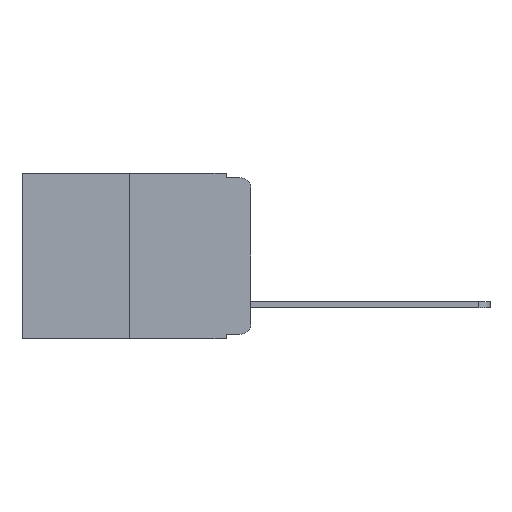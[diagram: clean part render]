
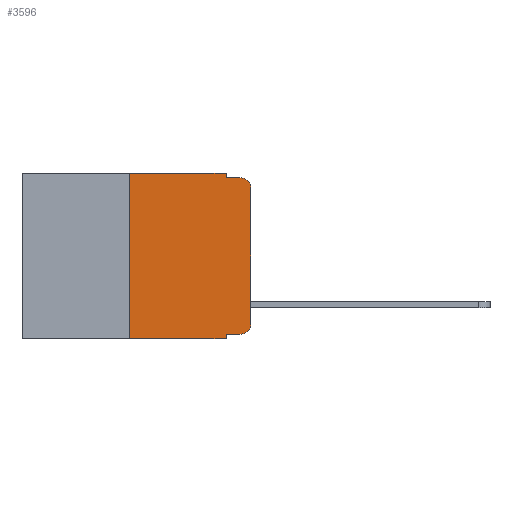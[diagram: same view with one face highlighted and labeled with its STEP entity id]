
A CAD part, left-side view. The second image highlights one B-rep face of the part: STEP entity #3596.
In plain terms, the highlighted planar face has unit normal (-1, 0, 0).
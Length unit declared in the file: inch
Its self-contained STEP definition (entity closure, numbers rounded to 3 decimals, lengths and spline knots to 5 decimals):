
#17 = CIRCLE ( 'NONE', #7517, 0.02 ) ;
#153 = CARTESIAN_POINT ( 'NONE',  ( 0., 0.051, -0.333 ) ) ;
#164 = CARTESIAN_POINT ( 'NONE',  ( 0., 0.473, 0. ) ) ;
#317 = EDGE_CURVE ( 'NONE', #16053, #17197, #1806, .T. ) ;
#400 = DIRECTION ( 'NONE',  ( -1., 0., 0. ) ) ;
#474 = EDGE_CURVE ( 'NONE', #8858, #903, #11412, .T. ) ;
#492 = CARTESIAN_POINT ( 'NONE',  ( 0., 0.051, -0.01 ) ) ;
#643 = VERTEX_POINT ( 'NONE', #5069 ) ;
#694 = CARTESIAN_POINT ( 'NONE',  ( 0., 0., 0. ) ) ;
#903 = VERTEX_POINT ( 'NONE', #4317 ) ;
#1048 = LINE ( 'NONE', #9050, #5649 ) ;
#1276 = EDGE_CURVE ( 'NONE', #903, #6998, #17, .T. ) ;
#1806 = LINE ( 'NONE', #12466, #5091 ) ;
#1963 = VECTOR ( 'NONE', #3531, 39.37008 ) ;
#2827 = ORIENTED_EDGE ( 'NONE', *, *, #474, .T. ) ;
#2914 = CARTESIAN_POINT ( 'NONE',  ( 0., 0.051, 0. ) ) ;
#3210 = DIRECTION ( 'NONE',  ( 0., 0., -1. ) ) ;
#3531 = DIRECTION ( 'NONE',  ( 0., 0., -1. ) ) ;
#3596 = ADVANCED_FACE ( 'NONE', ( #5192 ), #17017, .F. ) ;
#4317 = CARTESIAN_POINT ( 'NONE',  ( 0., 0., -0.03 ) ) ;
#4720 = ORIENTED_EDGE ( 'NONE', *, *, #8834, .T. ) ;
#4814 = CARTESIAN_POINT ( 'NONE',  ( 0., 0.02, -0.01 ) ) ;
#5069 = CARTESIAN_POINT ( 'NONE',  ( 0., 0.02, -0.333 ) ) ;
#5091 = VECTOR ( 'NONE', #14160, 39.37008 ) ;
#5192 = FACE_OUTER_BOUND ( 'NONE', #8830, .T. ) ;
#5333 = EDGE_CURVE ( 'NONE', #11239, #12072, #12685, .T. ) ;
#5520 = CARTESIAN_POINT ( 'NONE',  ( 0., 0.25, 0. ) ) ;
#5553 = VERTEX_POINT ( 'NONE', #153 ) ;
#5649 = VECTOR ( 'NONE', #6195, 39.37008 ) ;
#5858 = DIRECTION ( 'NONE',  ( 1., 0., 0. ) ) ;
#6097 = DIRECTION ( 'NONE',  ( 0., 0., 1. ) ) ;
#6195 = DIRECTION ( 'NONE',  ( 0., 0., -1. ) ) ;
#6376 = CIRCLE ( 'NONE', #9306, 0.02 ) ;
#6530 = EDGE_CURVE ( 'NONE', #5553, #17197, #1048, .T. ) ;
#6680 = VECTOR ( 'NONE', #7346, 39.37008 ) ;
#6871 = LINE ( 'NONE', #9982, #10804 ) ;
#6998 = VERTEX_POINT ( 'NONE', #4814 ) ;
#7221 = DIRECTION ( 'NONE',  ( 0., -1., 0. ) ) ;
#7275 = LINE ( 'NONE', #15207, #14508 ) ;
#7346 = DIRECTION ( 'NONE',  ( 0., -1., 0. ) ) ;
#7517 = AXIS2_PLACEMENT_3D ( 'NONE', #10187, #400, #3210 ) ;
#7597 = EDGE_CURVE ( 'NONE', #16053, #17313, #16533, .T. ) ;
#8536 = DIRECTION ( 'NONE',  ( 0., 0., -1. ) ) ;
#8585 = DIRECTION ( 'NONE',  ( 0., 0., -1. ) ) ;
#8830 = EDGE_LOOP ( 'NONE', ( #2827, #12749, #13470, #10991, #16631, #11613, #12989, #10913, #4720, #17436 ) ) ;
#8834 = EDGE_CURVE ( 'NONE', #5553, #643, #7275, .T. ) ;
#8858 = VERTEX_POINT ( 'NONE', #12462 ) ;
#9050 = CARTESIAN_POINT ( 'NONE',  ( 0., 0.051, 0. ) ) ;
#9155 = CARTESIAN_POINT ( 'NONE',  ( 0., 0.051, 0. ) ) ;
#9306 = AXIS2_PLACEMENT_3D ( 'NONE', #16670, #12716, #8536 ) ;
#9319 = DIRECTION ( 'NONE',  ( 0., 0., 1. ) ) ;
#9982 = CARTESIAN_POINT ( 'NONE',  ( 0., 0.473, 0. ) ) ;
#10187 = CARTESIAN_POINT ( 'NONE',  ( 0., 0.02, -0.03 ) ) ;
#10804 = VECTOR ( 'NONE', #7221, 39.37008 ) ;
#10913 = ORIENTED_EDGE ( 'NONE', *, *, #6530, .F. ) ;
#10991 = ORIENTED_EDGE ( 'NONE', *, *, #5333, .F. ) ;
#11034 = DIRECTION ( 'NONE',  ( 0., -1., 0. ) ) ;
#11048 = CARTESIAN_POINT ( 'NONE',  ( 0., 0.25, -0.343 ) ) ;
#11239 = VERTEX_POINT ( 'NONE', #2914 ) ;
#11412 = LINE ( 'NONE', #694, #17959 ) ;
#11613 = ORIENTED_EDGE ( 'NONE', *, *, #7597, .F. ) ;
#12072 = VERTEX_POINT ( 'NONE', #492 ) ;
#12462 = CARTESIAN_POINT ( 'NONE',  ( 0., 0., -0.313 ) ) ;
#12466 = CARTESIAN_POINT ( 'NONE',  ( 0., 0.473, -0.343 ) ) ;
#12685 = LINE ( 'NONE', #9155, #1963 ) ;
#12716 = DIRECTION ( 'NONE',  ( -1., 0., 0. ) ) ;
#12749 = ORIENTED_EDGE ( 'NONE', *, *, #1276, .T. ) ;
#12762 = EDGE_CURVE ( 'NONE', #643, #8858, #6376, .T. ) ;
#12798 = CARTESIAN_POINT ( 'NONE',  ( 0., 0.051, -0.01 ) ) ;
#12989 = ORIENTED_EDGE ( 'NONE', *, *, #317, .T. ) ;
#13283 = AXIS2_PLACEMENT_3D ( 'NONE', #164, #5858, #8585 ) ;
#13470 = ORIENTED_EDGE ( 'NONE', *, *, #16860, .F. ) ;
#14160 = DIRECTION ( 'NONE',  ( 0., -1., 0. ) ) ;
#14508 = VECTOR ( 'NONE', #11034, 39.37008 ) ;
#14574 = VECTOR ( 'NONE', #6097, 39.37008 ) ;
#15002 = LINE ( 'NONE', #12798, #6680 ) ;
#15207 = CARTESIAN_POINT ( 'NONE',  ( 0., 0.051, -0.333 ) ) ;
#15973 = CARTESIAN_POINT ( 'NONE',  ( 0., 0.25, 0. ) ) ;
#16053 = VERTEX_POINT ( 'NONE', #11048 ) ;
#16465 = CARTESIAN_POINT ( 'NONE',  ( 0., 0.051, -0.343 ) ) ;
#16533 = LINE ( 'NONE', #15973, #14574 ) ;
#16631 = ORIENTED_EDGE ( 'NONE', *, *, #17529, .F. ) ;
#16670 = CARTESIAN_POINT ( 'NONE',  ( 0., 0.02, -0.313 ) ) ;
#16860 = EDGE_CURVE ( 'NONE', #12072, #6998, #15002, .T. ) ;
#17017 = PLANE ( 'NONE',  #13283 ) ;
#17197 = VERTEX_POINT ( 'NONE', #16465 ) ;
#17313 = VERTEX_POINT ( 'NONE', #5520 ) ;
#17436 = ORIENTED_EDGE ( 'NONE', *, *, #12762, .T. ) ;
#17529 = EDGE_CURVE ( 'NONE', #17313, #11239, #6871, .T. ) ;
#17959 = VECTOR ( 'NONE', #9319, 39.37008 ) ;
